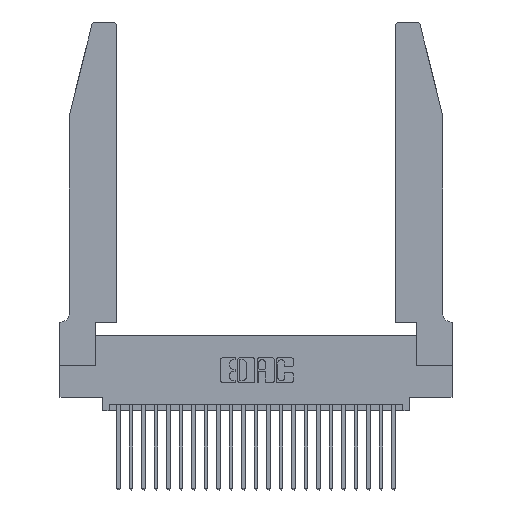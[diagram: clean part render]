
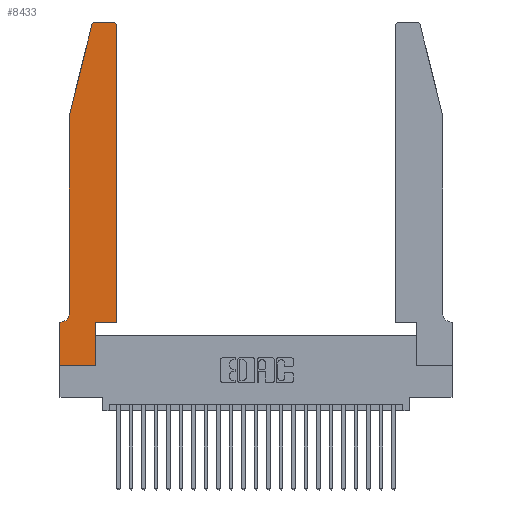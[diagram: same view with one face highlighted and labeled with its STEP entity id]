
A CAD part, top view. The second image highlights one B-rep face of the part: STEP entity #8433.
In plain terms, the highlighted planar face has unit normal (0, 0, 1).
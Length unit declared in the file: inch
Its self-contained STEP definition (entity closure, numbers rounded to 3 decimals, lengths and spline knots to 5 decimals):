
#120 = VERTEX_POINT ( 'NONE', #24487 ) ;
#603 = LINE ( 'NONE', #25040, #5391 ) ;
#1123 = ORIENTED_EDGE ( 'NONE', *, *, #21524, .T. ) ;
#1396 = AXIS2_PLACEMENT_3D ( 'NONE', #5766, #19518, #7818 ) ;
#1507 = DIRECTION ( 'NONE',  ( -1., 0., 0. ) ) ;
#1545 = CARTESIAN_POINT ( 'NONE',  ( 0.4205, 2.75, 0.37 ) ) ;
#1903 = ORIENTED_EDGE ( 'NONE', *, *, #23448, .T. ) ;
#1952 = VECTOR ( 'NONE', #7243, 39.37008 ) ;
#1970 = DIRECTION ( 'NONE',  ( 1., 0., 0. ) ) ;
#2218 = DIRECTION ( 'NONE',  ( 0., 0., 1. ) ) ;
#2727 = CARTESIAN_POINT ( 'NONE',  ( 0.4505, 0.35, 0.37 ) ) ;
#2810 = VERTEX_POINT ( 'NONE', #12743 ) ;
#2900 = VECTOR ( 'NONE', #14951, 39.37008 ) ;
#2955 = CARTESIAN_POINT ( 'NONE',  ( 0.4505, 0.35, 0.37 ) ) ;
#3008 = CARTESIAN_POINT ( 'NONE',  ( 0.0755, 0.35, 0.37 ) ) ;
#3009 = ORIENTED_EDGE ( 'NONE', *, *, #5122, .T. ) ;
#3077 = EDGE_CURVE ( 'NONE', #3590, #20963, #10572, .T. ) ;
#3246 = ORIENTED_EDGE ( 'NONE', *, *, #13178, .T. ) ;
#3590 = VERTEX_POINT ( 'NONE', #7895 ) ;
#3886 = DIRECTION ( 'NONE',  ( -0.239, -0.971, 0. ) ) ;
#4057 = EDGE_LOOP ( 'NONE', ( #3009, #9681, #17005, #13187, #19111, #12603, #23484, #1123, #3246, #25194, #1903, #11397 ) ) ;
#5122 = EDGE_CURVE ( 'NONE', #20696, #23727, #603, .T. ) ;
#5391 = VECTOR ( 'NONE', #1507, 39.37008 ) ;
#5766 = CARTESIAN_POINT ( 'NONE',  ( 0.0055, 0.42, 0.37 ) ) ;
#6052 = EDGE_CURVE ( 'NONE', #24093, #20696, #8282, .T. ) ;
#6073 = VERTEX_POINT ( 'NONE', #2727 ) ;
#6351 = PLANE ( 'NONE',  #14123 ) ;
#7218 = VERTEX_POINT ( 'NONE', #14788 ) ;
#7243 = DIRECTION ( 'NONE',  ( 0., 1., 0. ) ) ;
#7818 = DIRECTION ( 'NONE',  ( -1., 0., 0. ) ) ;
#7895 = CARTESIAN_POINT ( 'NONE',  ( 0.0755, 0.42, 0.37 ) ) ;
#8282 = CIRCLE ( 'NONE', #23052, 0.03 ) ;
#8433 = ADVANCED_FACE ( 'NONE', ( #24819 ), #6351, .T. ) ;
#8699 = CARTESIAN_POINT ( 'NONE',  ( 0.4505, 2.72, 0.37 ) ) ;
#8772 = DIRECTION ( 'NONE',  ( 0., 0., 1. ) ) ;
#9681 = ORIENTED_EDGE ( 'NONE', *, *, #14139, .T. ) ;
#10572 = CIRCLE ( 'NONE', #1396, 0.07 ) ;
#10715 = VECTOR ( 'NONE', #15510, 39.37008 ) ;
#10760 = CARTESIAN_POINT ( 'NONE',  ( 0.4205, 2.72, 0.37 ) ) ;
#11350 = LINE ( 'NONE', #24928, #10715 ) ;
#11397 = ORIENTED_EDGE ( 'NONE', *, *, #6052, .T. ) ;
#11460 = LINE ( 'NONE', #17785, #21105 ) ;
#11484 = CARTESIAN_POINT ( 'NONE',  ( 0., 0.35, 0.37 ) ) ;
#12258 = CARTESIAN_POINT ( 'NONE',  ( 0., 0.35, 0.37 ) ) ;
#12603 = ORIENTED_EDGE ( 'NONE', *, *, #22305, .T. ) ;
#12743 = CARTESIAN_POINT ( 'NONE',  ( 0.2865, 0.35, 0.37 ) ) ;
#12784 = DIRECTION ( 'NONE',  ( 1., 0., 0. ) ) ;
#13000 = CIRCLE ( 'NONE', #16770, 0.03 ) ;
#13001 = VECTOR ( 'NONE', #18834, 39.37008 ) ;
#13178 = EDGE_CURVE ( 'NONE', #21016, #2810, #24099, .T. ) ;
#13187 = ORIENTED_EDGE ( 'NONE', *, *, #22642, .T. ) ;
#13589 = LINE ( 'NONE', #2955, #2900 ) ;
#13744 = CARTESIAN_POINT ( 'NONE',  ( 0.284, 2.75, 0.37 ) ) ;
#13908 = VECTOR ( 'NONE', #3886, 39.37008 ) ;
#14123 = AXIS2_PLACEMENT_3D ( 'NONE', #12258, #8772, #22336 ) ;
#14139 = EDGE_CURVE ( 'NONE', #23727, #22196, #13000, .T. ) ;
#14250 = CARTESIAN_POINT ( 'NONE',  ( 0.284, 2.72, 0.37 ) ) ;
#14508 = VERTEX_POINT ( 'NONE', #11484 ) ;
#14619 = CARTESIAN_POINT ( 'NONE',  ( 0.2865, 0., 0.37 ) ) ;
#14788 = CARTESIAN_POINT ( 'NONE',  ( 0., 0., 0.37 ) ) ;
#14951 = DIRECTION ( 'NONE',  ( 0., 1., 0. ) ) ;
#15427 = LINE ( 'NONE', #16326, #24961 ) ;
#15510 = DIRECTION ( 'NONE',  ( 0., -1., 0. ) ) ;
#16190 = DIRECTION ( 'NONE',  ( 1., 0., 0. ) ) ;
#16326 = CARTESIAN_POINT ( 'NONE',  ( 0.0755, 2., 0.37 ) ) ;
#16770 = AXIS2_PLACEMENT_3D ( 'NONE', #14250, #2218, #16190 ) ;
#16939 = EDGE_CURVE ( 'NONE', #14508, #7218, #11350, .T. ) ;
#17005 = ORIENTED_EDGE ( 'NONE', *, *, #22490, .T. ) ;
#17785 = CARTESIAN_POINT ( 'NONE',  ( 0., 0., 0.37 ) ) ;
#18246 = DIRECTION ( 'NONE',  ( 0., -1., 0. ) ) ;
#18834 = DIRECTION ( 'NONE',  ( -1., 0., 0. ) ) ;
#19111 = ORIENTED_EDGE ( 'NONE', *, *, #3077, .T. ) ;
#19518 = DIRECTION ( 'NONE',  ( 0., 0., -1. ) ) ;
#19795 = VECTOR ( 'NONE', #24125, 39.37008 ) ;
#20696 = VERTEX_POINT ( 'NONE', #1545 ) ;
#20901 = CARTESIAN_POINT ( 'NONE',  ( 0.2865, 0.35, 0.37 ) ) ;
#20963 = VERTEX_POINT ( 'NONE', #22136 ) ;
#21016 = VERTEX_POINT ( 'NONE', #14619 ) ;
#21105 = VECTOR ( 'NONE', #1970, 39.37008 ) ;
#21524 = EDGE_CURVE ( 'NONE', #7218, #21016, #11460, .T. ) ;
#21577 = CARTESIAN_POINT ( 'NONE',  ( 0.0755, 2., 0.37 ) ) ;
#22136 = CARTESIAN_POINT ( 'NONE',  ( 0.0055, 0.35, 0.37 ) ) ;
#22196 = VERTEX_POINT ( 'NONE', #22263 ) ;
#22203 = CARTESIAN_POINT ( 'NONE',  ( 0.4505, 0.35, 0.37 ) ) ;
#22263 = CARTESIAN_POINT ( 'NONE',  ( 0.25487, 2.72718, 0.37 ) ) ;
#22305 = EDGE_CURVE ( 'NONE', #20963, #14508, #23185, .T. ) ;
#22336 = DIRECTION ( 'NONE',  ( 1., 0., 0. ) ) ;
#22490 = EDGE_CURVE ( 'NONE', #22196, #120, #24672, .T. ) ;
#22642 = EDGE_CURVE ( 'NONE', #120, #3590, #15427, .T. ) ;
#23052 = AXIS2_PLACEMENT_3D ( 'NONE', #10760, #24249, #12784 ) ;
#23185 = LINE ( 'NONE', #3008, #13001 ) ;
#23448 = EDGE_CURVE ( 'NONE', #6073, #24093, #13589, .T. ) ;
#23484 = ORIENTED_EDGE ( 'NONE', *, *, #16939, .T. ) ;
#23727 = VERTEX_POINT ( 'NONE', #13744 ) ;
#24093 = VERTEX_POINT ( 'NONE', #8699 ) ;
#24099 = LINE ( 'NONE', #20901, #1952 ) ;
#24125 = DIRECTION ( 'NONE',  ( 1., 0., 0. ) ) ;
#24249 = DIRECTION ( 'NONE',  ( 0., 0., 1. ) ) ;
#24487 = CARTESIAN_POINT ( 'NONE',  ( 0.0755, 2., 0.37 ) ) ;
#24672 = LINE ( 'NONE', #21577, #13908 ) ;
#24819 = FACE_OUTER_BOUND ( 'NONE', #4057, .T. ) ;
#24928 = CARTESIAN_POINT ( 'NONE',  ( 0., 0., 0.37 ) ) ;
#24961 = VECTOR ( 'NONE', #18246, 39.37008 ) ;
#25040 = CARTESIAN_POINT ( 'NONE',  ( 0.2605, 2.75, 0.37 ) ) ;
#25194 = ORIENTED_EDGE ( 'NONE', *, *, #25231, .T. ) ;
#25231 = EDGE_CURVE ( 'NONE', #2810, #6073, #25468, .T. ) ;
#25468 = LINE ( 'NONE', #22203, #19795 ) ;
